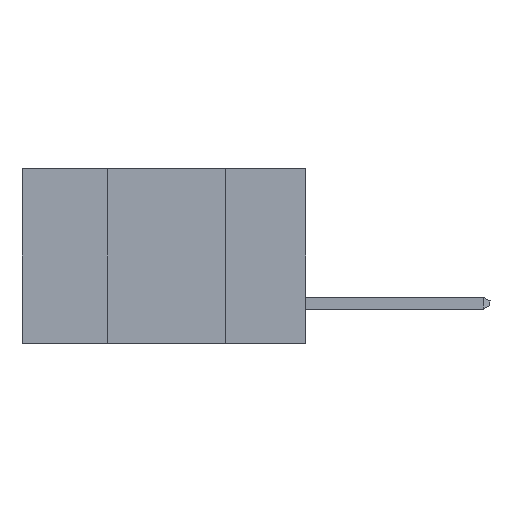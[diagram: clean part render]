
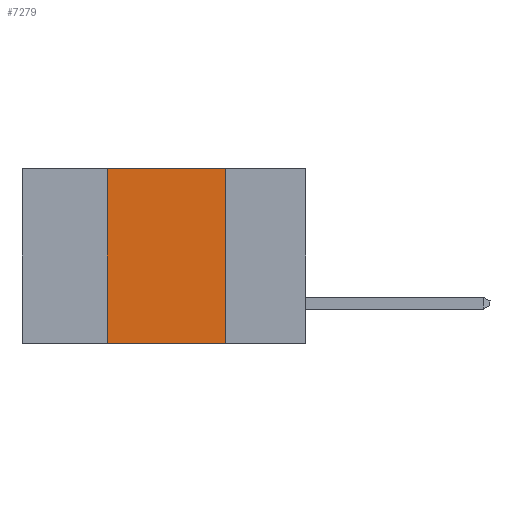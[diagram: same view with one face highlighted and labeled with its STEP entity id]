
A CAD part, left-side view. The second image highlights one B-rep face of the part: STEP entity #7279.
In plain terms, the highlighted planar face has unit normal (-1, 0, 0).
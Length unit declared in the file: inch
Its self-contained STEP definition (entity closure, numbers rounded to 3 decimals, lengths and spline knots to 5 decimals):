
#70 = LINE ( 'NONE', #839, #4778 ) ;
#107 = DIRECTION ( 'NONE',  ( 0., -1., 0. ) ) ;
#175 = VECTOR ( 'NONE', #264, 39.37008 ) ;
#264 = DIRECTION ( 'NONE',  ( 0., 0., -1. ) ) ;
#839 = CARTESIAN_POINT ( 'NONE',  ( 0., 0.6, -0.37 ) ) ;
#857 = VERTEX_POINT ( 'NONE', #7148 ) ;
#1034 = CARTESIAN_POINT ( 'NONE',  ( 0., 0.17, -0.37 ) ) ;
#1094 = CARTESIAN_POINT ( 'NONE',  ( 0., 0.6, 0. ) ) ;
#1334 = VECTOR ( 'NONE', #8873, 39.37008 ) ;
#1543 = ORIENTED_EDGE ( 'NONE', *, *, #5893, .F. ) ;
#1848 = PLANE ( 'NONE',  #1852 ) ;
#1852 = AXIS2_PLACEMENT_3D ( 'NONE', #1094, #3380, #6911 ) ;
#1976 = ORIENTED_EDGE ( 'NONE', *, *, #5126, .F. ) ;
#2274 = LINE ( 'NONE', #5281, #1334 ) ;
#2583 = VERTEX_POINT ( 'NONE', #9383 ) ;
#2679 = CARTESIAN_POINT ( 'NONE',  ( 0., 0.17, 0. ) ) ;
#3380 = DIRECTION ( 'NONE',  ( 1., 0., 0. ) ) ;
#4095 = FACE_OUTER_BOUND ( 'NONE', #5209, .T. ) ;
#4396 = VERTEX_POINT ( 'NONE', #4680 ) ;
#4680 = CARTESIAN_POINT ( 'NONE',  ( 0., 0.42, -0.37 ) ) ;
#4778 = VECTOR ( 'NONE', #5188, 39.37008 ) ;
#5126 = EDGE_CURVE ( 'NONE', #4396, #857, #2274, .T. ) ;
#5188 = DIRECTION ( 'NONE',  ( 0., -1., 0. ) ) ;
#5209 = EDGE_LOOP ( 'NONE', ( #1543, #5666, #1976, #8910 ) ) ;
#5281 = CARTESIAN_POINT ( 'NONE',  ( 0., 0.42, -0.37 ) ) ;
#5666 = ORIENTED_EDGE ( 'NONE', *, *, #6182, .F. ) ;
#5893 = EDGE_CURVE ( 'NONE', #7010, #2583, #8195, .T. ) ;
#6182 = EDGE_CURVE ( 'NONE', #857, #7010, #8041, .T. ) ;
#6457 = VECTOR ( 'NONE', #107, 39.37008 ) ;
#6911 = DIRECTION ( 'NONE',  ( 0., 0., -1. ) ) ;
#7010 = VERTEX_POINT ( 'NONE', #2679 ) ;
#7148 = CARTESIAN_POINT ( 'NONE',  ( 0., 0.42, 0. ) ) ;
#7279 = ADVANCED_FACE ( 'NONE', ( #4095 ), #1848, .F. ) ;
#7903 = CARTESIAN_POINT ( 'NONE',  ( 0., 0.6, 0. ) ) ;
#8041 = LINE ( 'NONE', #7903, #6457 ) ;
#8195 = LINE ( 'NONE', #1034, #175 ) ;
#8873 = DIRECTION ( 'NONE',  ( 0., 0., 1. ) ) ;
#8910 = ORIENTED_EDGE ( 'NONE', *, *, #9079, .T. ) ;
#9079 = EDGE_CURVE ( 'NONE', #4396, #2583, #70, .T. ) ;
#9383 = CARTESIAN_POINT ( 'NONE',  ( 0., 0.17, -0.37 ) ) ;
